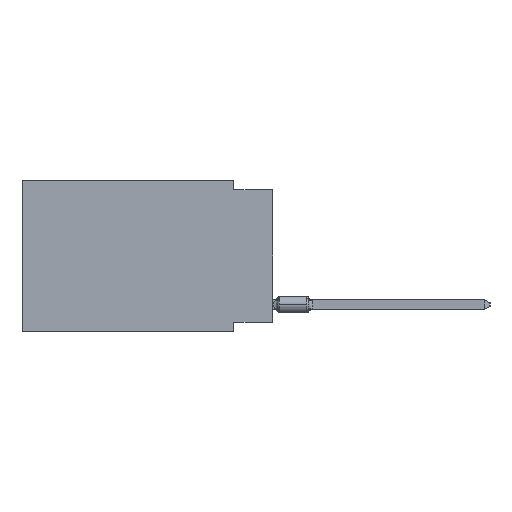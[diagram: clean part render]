
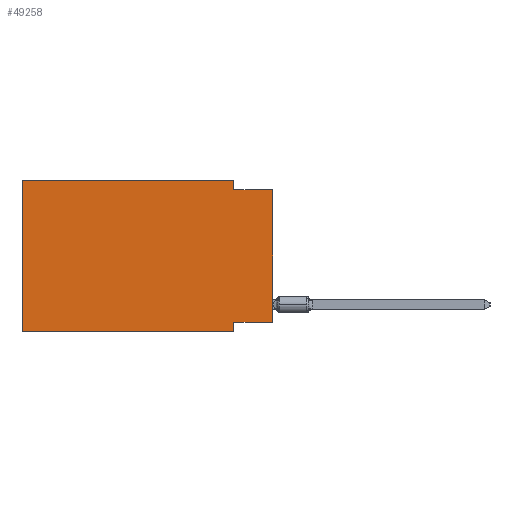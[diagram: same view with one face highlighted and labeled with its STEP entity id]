
A CAD part, left-side view. The second image highlights one B-rep face of the part: STEP entity #49258.
In plain terms, the highlighted planar face has unit normal (-1, 0, 0).
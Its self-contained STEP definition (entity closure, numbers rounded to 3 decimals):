
#190 = VERTEX_POINT ( 'NONE', #49242 ) ;
#217 = VECTOR ( 'NONE', #45536, 1000. ) ;
#530 = CARTESIAN_POINT ( 'NONE',  ( 0., 2.54, -9.271 ) ) ;
#1570 = LINE ( 'NONE', #13885, #24222 ) ;
#1881 = LINE ( 'NONE', #10174, #45650 ) ;
#2236 = CARTESIAN_POINT ( 'NONE',  ( 0., 2.54, -9.906 ) ) ;
#2486 = ORIENTED_EDGE ( 'NONE', *, *, #26392, .T. ) ;
#6435 = DIRECTION ( 'NONE',  ( 0., 0., -1. ) ) ;
#9105 = VERTEX_POINT ( 'NONE', #33360 ) ;
#9109 = ORIENTED_EDGE ( 'NONE', *, *, #44833, .F. ) ;
#10170 = ORIENTED_EDGE ( 'NONE', *, *, #54178, .F. ) ;
#10174 = CARTESIAN_POINT ( 'NONE',  ( 0., 16.383, 0. ) ) ;
#11031 = CARTESIAN_POINT ( 'NONE',  ( 0., 0., -0.635 ) ) ;
#12489 = EDGE_CURVE ( 'NONE', #43566, #25299, #55465, .T. ) ;
#13389 = ORIENTED_EDGE ( 'NONE', *, *, #18874, .F. ) ;
#13885 = CARTESIAN_POINT ( 'NONE',  ( 0., 2.54, 0. ) ) ;
#15329 = CARTESIAN_POINT ( 'NONE',  ( 0., 0., -9.271 ) ) ;
#16199 = ORIENTED_EDGE ( 'NONE', *, *, #50207, .F. ) ;
#18139 = FACE_OUTER_BOUND ( 'NONE', #34117, .T. ) ;
#18621 = DIRECTION ( 'NONE',  ( 0., 1., 0. ) ) ;
#18874 = EDGE_CURVE ( 'NONE', #19521, #26497, #21385, .T. ) ;
#19482 = CARTESIAN_POINT ( 'NONE',  ( 0., 16.383, 0. ) ) ;
#19521 = VERTEX_POINT ( 'NONE', #23572 ) ;
#19716 = VECTOR ( 'NONE', #18621, 1000. ) ;
#20287 = CARTESIAN_POINT ( 'NONE',  ( 0., 2.54, 0. ) ) ;
#21385 = LINE ( 'NONE', #55179, #43694 ) ;
#23572 = CARTESIAN_POINT ( 'NONE',  ( 0., 16.383, 0. ) ) ;
#24025 = DIRECTION ( 'NONE',  ( 0., -1., 0. ) ) ;
#24222 = VECTOR ( 'NONE', #6435, 1000. ) ;
#25299 = VERTEX_POINT ( 'NONE', #2236 ) ;
#26146 = VECTOR ( 'NONE', #55011, 1000. ) ;
#26392 = EDGE_CURVE ( 'NONE', #35130, #25299, #49234, .T. ) ;
#26497 = VERTEX_POINT ( 'NONE', #20287 ) ;
#27218 = CARTESIAN_POINT ( 'NONE',  ( 0., 0., -9.271 ) ) ;
#27354 = DIRECTION ( 'NONE',  ( 0., 0., 1. ) ) ;
#28062 = CARTESIAN_POINT ( 'NONE',  ( 0., 2.54, -9.906 ) ) ;
#28389 = CARTESIAN_POINT ( 'NONE',  ( 0., 0., 0. ) ) ;
#29603 = ORIENTED_EDGE ( 'NONE', *, *, #40956, .F. ) ;
#29622 = DIRECTION ( 'NONE',  ( 0., -1., 0. ) ) ;
#31033 = DIRECTION ( 'NONE',  ( 0., 0., -1. ) ) ;
#32648 = DIRECTION ( 'NONE',  ( 1., 0., 0. ) ) ;
#33360 = CARTESIAN_POINT ( 'NONE',  ( 0., 2.54, -0.635 ) ) ;
#34117 = EDGE_LOOP ( 'NONE', ( #44001, #16199, #10170, #13389, #29603, #2486, #50239, #9109 ) ) ;
#35130 = VERTEX_POINT ( 'NONE', #52702 ) ;
#37193 = CARTESIAN_POINT ( 'NONE',  ( 0., 16.383, -9.906 ) ) ;
#40956 = EDGE_CURVE ( 'NONE', #35130, #19521, #1881, .T. ) ;
#41977 = AXIS2_PLACEMENT_3D ( 'NONE', #19482, #32648, #31033 ) ;
#42560 = DIRECTION ( 'NONE',  ( 0., -1., 0. ) ) ;
#43566 = VERTEX_POINT ( 'NONE', #530 ) ;
#43694 = VECTOR ( 'NONE', #42560, 1000. ) ;
#44001 = ORIENTED_EDGE ( 'NONE', *, *, #55495, .T. ) ;
#44833 = EDGE_CURVE ( 'NONE', #51000, #43566, #52725, .T. ) ;
#45291 = LINE ( 'NONE', #28389, #26146 ) ;
#45536 = DIRECTION ( 'NONE',  ( 0., 0., -1. ) ) ;
#45650 = VECTOR ( 'NONE', #27354, 1000. ) ;
#45820 = PLANE ( 'NONE',  #41977 ) ;
#49234 = LINE ( 'NONE', #37193, #53144 ) ;
#49242 = CARTESIAN_POINT ( 'NONE',  ( 0., 0., -0.635 ) ) ;
#49258 = ADVANCED_FACE ( 'NONE', ( #18139 ), #45820, .F. ) ;
#50207 = EDGE_CURVE ( 'NONE', #9105, #190, #50253, .T. ) ;
#50239 = ORIENTED_EDGE ( 'NONE', *, *, #12489, .F. ) ;
#50253 = LINE ( 'NONE', #11031, #54353 ) ;
#51000 = VERTEX_POINT ( 'NONE', #15329 ) ;
#52702 = CARTESIAN_POINT ( 'NONE',  ( 0., 16.383, -9.906 ) ) ;
#52725 = LINE ( 'NONE', #27218, #19716 ) ;
#53144 = VECTOR ( 'NONE', #24025, 1000. ) ;
#54178 = EDGE_CURVE ( 'NONE', #26497, #9105, #1570, .T. ) ;
#54353 = VECTOR ( 'NONE', #29622, 1000. ) ;
#55011 = DIRECTION ( 'NONE',  ( 0., 0., 1. ) ) ;
#55179 = CARTESIAN_POINT ( 'NONE',  ( 0., 16.383, 0. ) ) ;
#55465 = LINE ( 'NONE', #28062, #217 ) ;
#55495 = EDGE_CURVE ( 'NONE', #51000, #190, #45291, .T. ) ;
